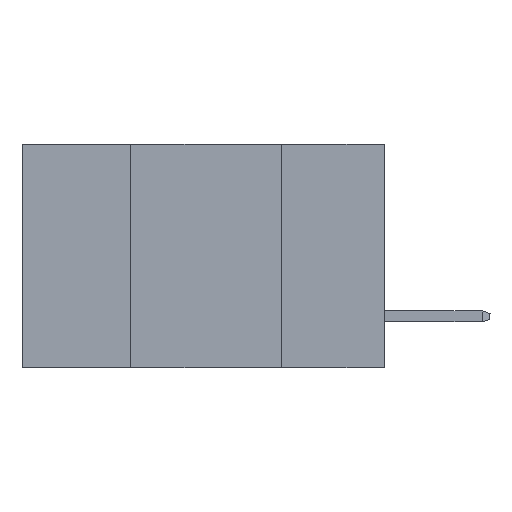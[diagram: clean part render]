
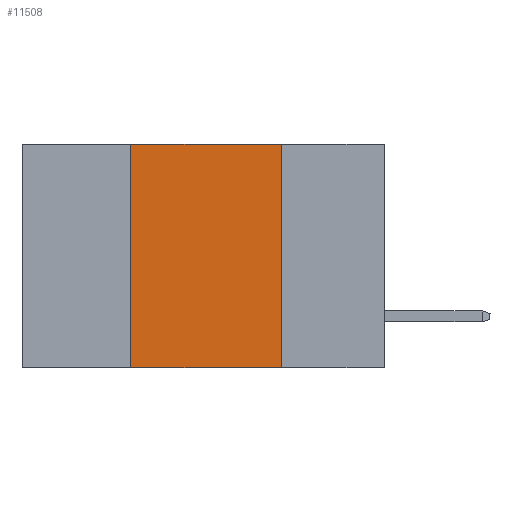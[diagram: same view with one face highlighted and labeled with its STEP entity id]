
A CAD part, left-side view. The second image highlights one B-rep face of the part: STEP entity #11508.
In plain terms, the highlighted planar face has unit normal (-1, 0, 0).
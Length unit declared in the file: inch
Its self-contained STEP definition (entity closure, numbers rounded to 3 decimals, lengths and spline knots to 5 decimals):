
#365 = CARTESIAN_POINT ( 'NONE',  ( 0., 0.6, -0.37 ) ) ;
#948 = FACE_OUTER_BOUND ( 'NONE', #17165, .T. ) ;
#3276 = DIRECTION ( 'NONE',  ( 1., 0., 0. ) ) ;
#3845 = DIRECTION ( 'NONE',  ( 0., -1., 0. ) ) ;
#5161 = VECTOR ( 'NONE', #3845, 39.37008 ) ;
#5379 = LINE ( 'NONE', #10118, #15099 ) ;
#5445 = CARTESIAN_POINT ( 'NONE',  ( 0., 0.17, 0. ) ) ;
#5490 = DIRECTION ( 'NONE',  ( 0., 0., 1. ) ) ;
#6689 = EDGE_CURVE ( 'NONE', #12720, #12591, #10030, .T. ) ;
#7274 = ORIENTED_EDGE ( 'NONE', *, *, #6689, .F. ) ;
#7710 = CARTESIAN_POINT ( 'NONE',  ( 0., 0.42, -0.37 ) ) ;
#7924 = CARTESIAN_POINT ( 'NONE',  ( 0., 0.6, 0. ) ) ;
#8881 = EDGE_CURVE ( 'NONE', #12720, #15844, #10066, .T. ) ;
#9918 = ORIENTED_EDGE ( 'NONE', *, *, #13057, .F. ) ;
#10030 = LINE ( 'NONE', #18227, #10704 ) ;
#10066 = LINE ( 'NONE', #365, #16348 ) ;
#10118 = CARTESIAN_POINT ( 'NONE',  ( 0., 0.17, -0.37 ) ) ;
#10704 = VECTOR ( 'NONE', #5490, 39.37008 ) ;
#11508 = ADVANCED_FACE ( 'NONE', ( #948 ), #14143, .F. ) ;
#11740 = DIRECTION ( 'NONE',  ( 0., -1., 0. ) ) ;
#12568 = LINE ( 'NONE', #14149, #5161 ) ;
#12591 = VERTEX_POINT ( 'NONE', #14620 ) ;
#12670 = DIRECTION ( 'NONE',  ( 0., 0., -1. ) ) ;
#12720 = VERTEX_POINT ( 'NONE', #7710 ) ;
#13057 = EDGE_CURVE ( 'NONE', #18493, #15844, #5379, .T. ) ;
#14143 = PLANE ( 'NONE',  #19387 ) ;
#14149 = CARTESIAN_POINT ( 'NONE',  ( 0., 0.6, 0. ) ) ;
#14620 = CARTESIAN_POINT ( 'NONE',  ( 0., 0.42, 0. ) ) ;
#15099 = VECTOR ( 'NONE', #16545, 39.37008 ) ;
#15844 = VERTEX_POINT ( 'NONE', #19535 ) ;
#16348 = VECTOR ( 'NONE', #11740, 39.37008 ) ;
#16545 = DIRECTION ( 'NONE',  ( 0., 0., -1. ) ) ;
#17165 = EDGE_LOOP ( 'NONE', ( #9918, #17777, #7274, #18890 ) ) ;
#17777 = ORIENTED_EDGE ( 'NONE', *, *, #20737, .F. ) ;
#18227 = CARTESIAN_POINT ( 'NONE',  ( 0., 0.42, -0.37 ) ) ;
#18493 = VERTEX_POINT ( 'NONE', #5445 ) ;
#18890 = ORIENTED_EDGE ( 'NONE', *, *, #8881, .T. ) ;
#19387 = AXIS2_PLACEMENT_3D ( 'NONE', #7924, #3276, #12670 ) ;
#19535 = CARTESIAN_POINT ( 'NONE',  ( 0., 0.17, -0.37 ) ) ;
#20737 = EDGE_CURVE ( 'NONE', #12591, #18493, #12568, .T. ) ;
